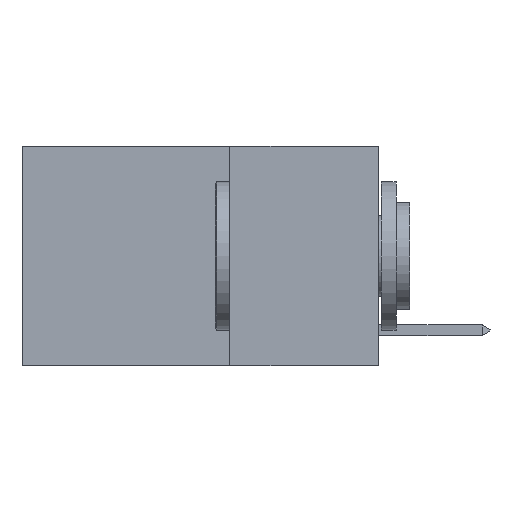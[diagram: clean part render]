
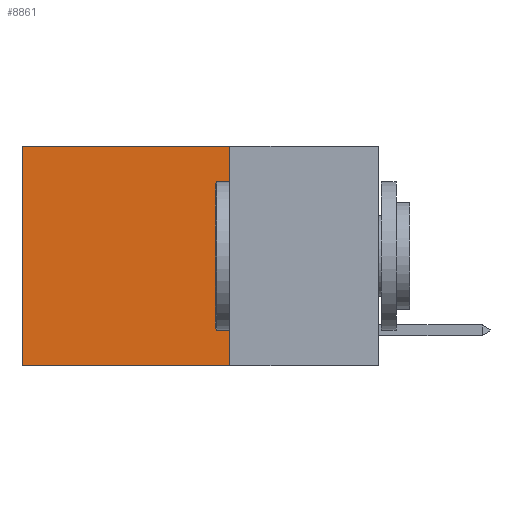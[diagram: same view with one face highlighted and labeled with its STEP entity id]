
A CAD part, left-side view. The second image highlights one B-rep face of the part: STEP entity #8861.
In plain terms, the highlighted planar face has unit normal (-1, 0, 0).
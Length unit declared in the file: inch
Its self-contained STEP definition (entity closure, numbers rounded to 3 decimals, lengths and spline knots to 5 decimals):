
#251 = CARTESIAN_POINT ( 'NONE',  ( 0.2625, 0.6, -0.37 ) ) ;
#387 = CARTESIAN_POINT ( 'NONE',  ( 0.2625, 0.25, 0. ) ) ;
#982 = DIRECTION ( 'NONE',  ( 0., 1., 0. ) ) ;
#1271 = EDGE_CURVE ( 'NONE', #11474, #14383, #10516, .T. ) ;
#1309 = VECTOR ( 'NONE', #4366, 39.37008 ) ;
#1462 = CARTESIAN_POINT ( 'NONE',  ( 0.2625, 0.25, 0. ) ) ;
#1627 = ORIENTED_EDGE ( 'NONE', *, *, #12731, .T. ) ;
#2074 = LINE ( 'NONE', #5466, #11386 ) ;
#2655 = EDGE_CURVE ( 'NONE', #11474, #5998, #12263, .T. ) ;
#2811 = ORIENTED_EDGE ( 'NONE', *, *, #8234, .F. ) ;
#3250 = AXIS2_PLACEMENT_3D ( 'NONE', #1462, #12768, #6997 ) ;
#3915 = LINE ( 'NONE', #7290, #9992 ) ;
#4366 = DIRECTION ( 'NONE',  ( 0., 1., 0. ) ) ;
#5420 = VERTEX_POINT ( 'NONE', #251 ) ;
#5466 = CARTESIAN_POINT ( 'NONE',  ( 0.2625, 0.25, -0.37 ) ) ;
#5971 = CARTESIAN_POINT ( 'NONE',  ( 0.2625, 0.6, 0. ) ) ;
#5998 = VERTEX_POINT ( 'NONE', #5971 ) ;
#6997 = DIRECTION ( 'NONE',  ( 0., 0., -1. ) ) ;
#7203 = EDGE_LOOP ( 'NONE', ( #1627, #2811, #11130, #14282 ) ) ;
#7290 = CARTESIAN_POINT ( 'NONE',  ( 0.2625, 0.6, 0. ) ) ;
#8234 = EDGE_CURVE ( 'NONE', #14383, #5420, #2074, .T. ) ;
#8385 = FACE_OUTER_BOUND ( 'NONE', #7203, .T. ) ;
#8861 = ADVANCED_FACE ( 'NONE', ( #8385 ), #11576, .F. ) ;
#9665 = DIRECTION ( 'NONE',  ( 0., 0., -1. ) ) ;
#9797 = CARTESIAN_POINT ( 'NONE',  ( 0.2625, 0.25, 0. ) ) ;
#9992 = VECTOR ( 'NONE', #9665, 39.37008 ) ;
#10516 = LINE ( 'NONE', #387, #12615 ) ;
#10668 = CARTESIAN_POINT ( 'NONE',  ( 0.2625, 0.25, -0.37 ) ) ;
#11130 = ORIENTED_EDGE ( 'NONE', *, *, #1271, .F. ) ;
#11386 = VECTOR ( 'NONE', #982, 39.37008 ) ;
#11474 = VERTEX_POINT ( 'NONE', #9797 ) ;
#11576 = PLANE ( 'NONE',  #3250 ) ;
#12263 = LINE ( 'NONE', #13341, #1309 ) ;
#12615 = VECTOR ( 'NONE', #12650, 39.37008 ) ;
#12650 = DIRECTION ( 'NONE',  ( 0., 0., -1. ) ) ;
#12731 = EDGE_CURVE ( 'NONE', #5998, #5420, #3915, .T. ) ;
#12768 = DIRECTION ( 'NONE',  ( 1., 0., 0. ) ) ;
#13341 = CARTESIAN_POINT ( 'NONE',  ( 0.2625, 0.25, 0. ) ) ;
#14282 = ORIENTED_EDGE ( 'NONE', *, *, #2655, .T. ) ;
#14383 = VERTEX_POINT ( 'NONE', #10668 ) ;
